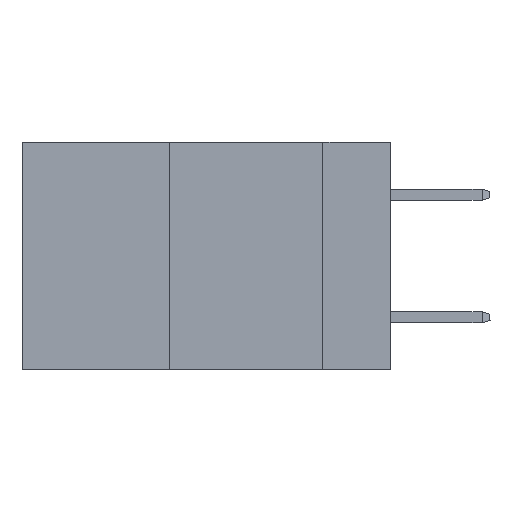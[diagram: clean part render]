
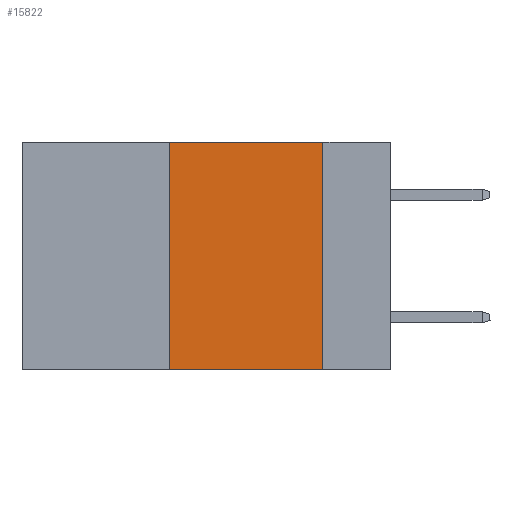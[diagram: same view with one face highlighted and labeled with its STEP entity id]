
A CAD part, left-side view. The second image highlights one B-rep face of the part: STEP entity #15822.
In plain terms, the highlighted planar face has unit normal (-1, 0, 0).
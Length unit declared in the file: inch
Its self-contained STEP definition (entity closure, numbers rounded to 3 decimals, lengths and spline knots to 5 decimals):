
#390 = ORIENTED_EDGE ( 'NONE', *, *, #18237, .F. ) ;
#1687 = EDGE_LOOP ( 'NONE', ( #15448, #390, #3386, #26951 ) ) ;
#1899 = VERTEX_POINT ( 'NONE', #24850 ) ;
#2170 = CARTESIAN_POINT ( 'NONE',  ( 0., 0.11, 0. ) ) ;
#2177 = CARTESIAN_POINT ( 'NONE',  ( 0., 0.36, -0.37 ) ) ;
#2654 = AXIS2_PLACEMENT_3D ( 'NONE', #12545, #17444, #3050 ) ;
#3050 = DIRECTION ( 'NONE',  ( 0., 0., -1. ) ) ;
#3386 = ORIENTED_EDGE ( 'NONE', *, *, #16896, .F. ) ;
#3553 = CARTESIAN_POINT ( 'NONE',  ( 0., 0.36, 0. ) ) ;
#3854 = CARTESIAN_POINT ( 'NONE',  ( 0., 0.11, 0. ) ) ;
#4055 = VECTOR ( 'NONE', #14007, 39.37008 ) ;
#7555 = PLANE ( 'NONE',  #2654 ) ;
#7891 = LINE ( 'NONE', #3553, #20769 ) ;
#8199 = EDGE_CURVE ( 'NONE', #22505, #1899, #24756, .T. ) ;
#8406 = DIRECTION ( 'NONE',  ( 0., -1., 0. ) ) ;
#9329 = VECTOR ( 'NONE', #18257, 39.37008 ) ;
#9605 = CARTESIAN_POINT ( 'NONE',  ( 0., 0.6, -0.37 ) ) ;
#10310 = VERTEX_POINT ( 'NONE', #30674 ) ;
#10855 = VECTOR ( 'NONE', #8406, 39.37008 ) ;
#11189 = LINE ( 'NONE', #3854, #9329 ) ;
#12545 = CARTESIAN_POINT ( 'NONE',  ( 0., 0.6, 0. ) ) ;
#13617 = CARTESIAN_POINT ( 'NONE',  ( 0., 0.6, 0. ) ) ;
#14007 = DIRECTION ( 'NONE',  ( 0., -1., 0. ) ) ;
#14121 = VERTEX_POINT ( 'NONE', #2170 ) ;
#15448 = ORIENTED_EDGE ( 'NONE', *, *, #18767, .F. ) ;
#15822 = ADVANCED_FACE ( 'NONE', ( #22333 ), #7555, .F. ) ;
#16896 = EDGE_CURVE ( 'NONE', #22505, #10310, #7891, .T. ) ;
#17444 = DIRECTION ( 'NONE',  ( 1., 0., 0. ) ) ;
#18237 = EDGE_CURVE ( 'NONE', #10310, #14121, #22182, .T. ) ;
#18257 = DIRECTION ( 'NONE',  ( 0., 0., -1. ) ) ;
#18767 = EDGE_CURVE ( 'NONE', #14121, #1899, #11189, .T. ) ;
#20769 = VECTOR ( 'NONE', #23305, 39.37008 ) ;
#22182 = LINE ( 'NONE', #13617, #10855 ) ;
#22333 = FACE_OUTER_BOUND ( 'NONE', #1687, .T. ) ;
#22505 = VERTEX_POINT ( 'NONE', #2177 ) ;
#23305 = DIRECTION ( 'NONE',  ( 0., 0., 1. ) ) ;
#24756 = LINE ( 'NONE', #9605, #4055 ) ;
#24850 = CARTESIAN_POINT ( 'NONE',  ( 0., 0.11, -0.37 ) ) ;
#26951 = ORIENTED_EDGE ( 'NONE', *, *, #8199, .T. ) ;
#30674 = CARTESIAN_POINT ( 'NONE',  ( 0., 0.36, 0. ) ) ;
